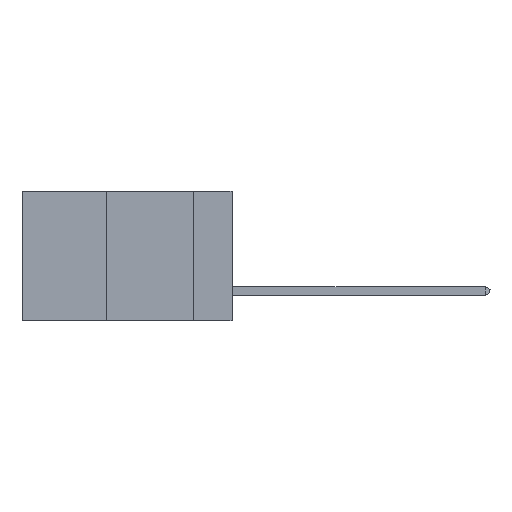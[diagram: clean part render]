
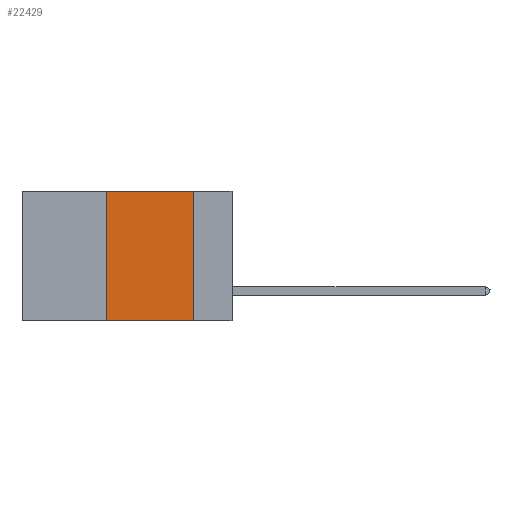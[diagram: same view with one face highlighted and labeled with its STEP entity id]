
A CAD part, left-side view. The second image highlights one B-rep face of the part: STEP entity #22429.
In plain terms, the highlighted planar face has unit normal (-1, 0, 0).
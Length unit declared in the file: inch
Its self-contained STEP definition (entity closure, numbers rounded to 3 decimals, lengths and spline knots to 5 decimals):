
#2313 = CARTESIAN_POINT ( 'NONE',  ( 0., 0.36, -0.37 ) ) ;
#2585 = FACE_OUTER_BOUND ( 'NONE', #24346, .T. ) ;
#2850 = LINE ( 'NONE', #11089, #17943 ) ;
#3231 = EDGE_CURVE ( 'NONE', #8928, #38914, #23991, .T. ) ;
#3284 = CARTESIAN_POINT ( 'NONE',  ( 0., 0.6, 0. ) ) ;
#4240 = DIRECTION ( 'NONE',  ( 0., -1., 0. ) ) ;
#5440 = DIRECTION ( 'NONE',  ( 0., 0., -1. ) ) ;
#6418 = DIRECTION ( 'NONE',  ( 0., 0., -1. ) ) ;
#7683 = CARTESIAN_POINT ( 'NONE',  ( 0., 0.6, 0. ) ) ;
#8761 = LINE ( 'NONE', #28266, #32560 ) ;
#8928 = VERTEX_POINT ( 'NONE', #22303 ) ;
#11089 = CARTESIAN_POINT ( 'NONE',  ( 0., 0.6, -0.37 ) ) ;
#11407 = VECTOR ( 'NONE', #5440, 39.37008 ) ;
#15626 = VERTEX_POINT ( 'NONE', #19711 ) ;
#15731 = PLANE ( 'NONE',  #38578 ) ;
#17328 = DIRECTION ( 'NONE',  ( 0., -1., 0. ) ) ;
#17943 = VECTOR ( 'NONE', #17328, 39.37008 ) ;
#18858 = ORIENTED_EDGE ( 'NONE', *, *, #27484, .F. ) ;
#19711 = CARTESIAN_POINT ( 'NONE',  ( 0., 0.36, 0. ) ) ;
#19779 = VERTEX_POINT ( 'NONE', #2313 ) ;
#21036 = LINE ( 'NONE', #7683, #34135 ) ;
#22303 = CARTESIAN_POINT ( 'NONE',  ( 0., 0.11, 0. ) ) ;
#22429 = ADVANCED_FACE ( 'NONE', ( #2585 ), #15731, .F. ) ;
#23991 = LINE ( 'NONE', #35026, #11407 ) ;
#24346 = EDGE_LOOP ( 'NONE', ( #27790, #25670, #18858, #38752 ) ) ;
#25053 = DIRECTION ( 'NONE',  ( 1., 0., 0. ) ) ;
#25670 = ORIENTED_EDGE ( 'NONE', *, *, #28801, .F. ) ;
#27484 = EDGE_CURVE ( 'NONE', #19779, #15626, #8761, .T. ) ;
#27790 = ORIENTED_EDGE ( 'NONE', *, *, #3231, .F. ) ;
#28266 = CARTESIAN_POINT ( 'NONE',  ( 0., 0.36, 0. ) ) ;
#28801 = EDGE_CURVE ( 'NONE', #15626, #8928, #21036, .T. ) ;
#29086 = DIRECTION ( 'NONE',  ( 0., 0., 1. ) ) ;
#32560 = VECTOR ( 'NONE', #29086, 39.37008 ) ;
#34135 = VECTOR ( 'NONE', #4240, 39.37008 ) ;
#35026 = CARTESIAN_POINT ( 'NONE',  ( 0., 0.11, 0. ) ) ;
#35611 = CARTESIAN_POINT ( 'NONE',  ( 0., 0.11, -0.37 ) ) ;
#37158 = EDGE_CURVE ( 'NONE', #19779, #38914, #2850, .T. ) ;
#38578 = AXIS2_PLACEMENT_3D ( 'NONE', #3284, #25053, #6418 ) ;
#38752 = ORIENTED_EDGE ( 'NONE', *, *, #37158, .T. ) ;
#38914 = VERTEX_POINT ( 'NONE', #35611 ) ;
